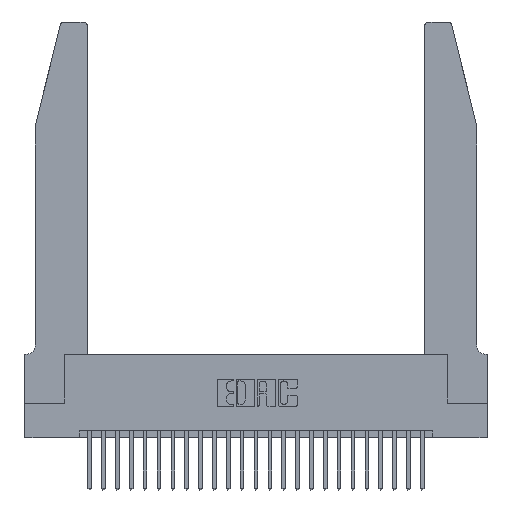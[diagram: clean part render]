
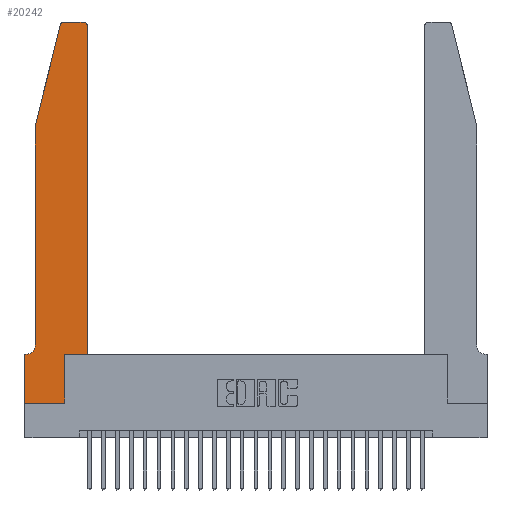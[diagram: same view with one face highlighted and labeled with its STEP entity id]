
A CAD part, top view. The second image highlights one B-rep face of the part: STEP entity #20242.
In plain terms, the highlighted planar face has unit normal (0, 0, 1).
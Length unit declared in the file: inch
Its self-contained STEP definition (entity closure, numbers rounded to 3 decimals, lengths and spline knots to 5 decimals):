
#42 = VECTOR ( 'NONE', #10206, 39.37008 ) ;
#264 = EDGE_CURVE ( 'NONE', #20774, #3971, #15840, .T. ) ;
#722 = FACE_OUTER_BOUND ( 'NONE', #21605, .T. ) ;
#1321 = VERTEX_POINT ( 'NONE', #15586 ) ;
#1489 = ORIENTED_EDGE ( 'NONE', *, *, #1849, .T. ) ;
#1694 = CARTESIAN_POINT ( 'NONE',  ( 0.0755, 0.42, 0.37 ) ) ;
#1849 = EDGE_CURVE ( 'NONE', #12343, #19882, #25817, .T. ) ;
#2294 = VECTOR ( 'NONE', #11618, 39.37008 ) ;
#3103 = DIRECTION ( 'NONE',  ( -0.239, -0.971, 0. ) ) ;
#3318 = ORIENTED_EDGE ( 'NONE', *, *, #16579, .T. ) ;
#3641 = PLANE ( 'NONE',  #5466 ) ;
#3971 = VERTEX_POINT ( 'NONE', #19977 ) ;
#4010 = DIRECTION ( 'NONE',  ( 0., 0., -1. ) ) ;
#4791 = DIRECTION ( 'NONE',  ( 0., 0., 1. ) ) ;
#4802 = EDGE_CURVE ( 'NONE', #21981, #8724, #15599, .T. ) ;
#4839 = VECTOR ( 'NONE', #3103, 39.37008 ) ;
#5466 = AXIS2_PLACEMENT_3D ( 'NONE', #18116, #5812, #20136 ) ;
#5775 = CARTESIAN_POINT ( 'NONE',  ( 0.2605, 2.75, 0.37 ) ) ;
#5780 = CARTESIAN_POINT ( 'NONE',  ( 0.25487, 2.72718, 0.37 ) ) ;
#5812 = DIRECTION ( 'NONE',  ( 0., 0., 1. ) ) ;
#5871 = EDGE_CURVE ( 'NONE', #24261, #24541, #8720, .T. ) ;
#5968 = DIRECTION ( 'NONE',  ( 0., -1., 0. ) ) ;
#6726 = CARTESIAN_POINT ( 'NONE',  ( 0.2865, 0.35, 0.37 ) ) ;
#6955 = EDGE_CURVE ( 'NONE', #3971, #21981, #16311, .T. ) ;
#7333 = EDGE_CURVE ( 'NONE', #25424, #12343, #23529, .T. ) ;
#7605 = CARTESIAN_POINT ( 'NONE',  ( 0.4205, 2.72, 0.37 ) ) ;
#8321 = DIRECTION ( 'NONE',  ( 0., -1., 0. ) ) ;
#8660 = CARTESIAN_POINT ( 'NONE',  ( 0.2865, 0., 0.37 ) ) ;
#8720 = CIRCLE ( 'NONE', #15561, 0.03 ) ;
#8724 = VERTEX_POINT ( 'NONE', #15977 ) ;
#8924 = AXIS2_PLACEMENT_3D ( 'NONE', #17145, #4791, #19156 ) ;
#9358 = VECTOR ( 'NONE', #16210, 39.37008 ) ;
#9700 = DIRECTION ( 'NONE',  ( 1., 0., 0. ) ) ;
#9787 = LINE ( 'NONE', #10392, #19938 ) ;
#10111 = EDGE_CURVE ( 'NONE', #20518, #25424, #9787, .T. ) ;
#10206 = DIRECTION ( 'NONE',  ( 0., 1., 0. ) ) ;
#10392 = CARTESIAN_POINT ( 'NONE',  ( 0., 0., 0.37 ) ) ;
#10727 = LINE ( 'NONE', #22314, #42 ) ;
#10774 = ORIENTED_EDGE ( 'NONE', *, *, #264, .T. ) ;
#11618 = DIRECTION ( 'NONE',  ( 1., 0., 0. ) ) ;
#12009 = VECTOR ( 'NONE', #25819, 39.37008 ) ;
#12221 = CARTESIAN_POINT ( 'NONE',  ( 0.2865, 0.35, 0.37 ) ) ;
#12343 = VERTEX_POINT ( 'NONE', #8660 ) ;
#12423 = CARTESIAN_POINT ( 'NONE',  ( 0.4505, 2.72, 0.37 ) ) ;
#12628 = LINE ( 'NONE', #23805, #12009 ) ;
#13145 = ORIENTED_EDGE ( 'NONE', *, *, #10111, .T. ) ;
#13219 = CARTESIAN_POINT ( 'NONE',  ( 0.4505, 0.35, 0.37 ) ) ;
#13655 = ORIENTED_EDGE ( 'NONE', *, *, #5871, .T. ) ;
#15008 = ORIENTED_EDGE ( 'NONE', *, *, #15850, .T. ) ;
#15404 = LINE ( 'NONE', #26222, #9358 ) ;
#15561 = AXIS2_PLACEMENT_3D ( 'NONE', #7605, #21805, #9700 ) ;
#15586 = CARTESIAN_POINT ( 'NONE',  ( 0.284, 2.75, 0.37 ) ) ;
#15599 = CIRCLE ( 'NONE', #22468, 0.07 ) ;
#15840 = LINE ( 'NONE', #24064, #4839 ) ;
#15850 = EDGE_CURVE ( 'NONE', #24541, #1321, #22457, .T. ) ;
#15977 = CARTESIAN_POINT ( 'NONE',  ( 0.0055, 0.35, 0.37 ) ) ;
#16210 = DIRECTION ( 'NONE',  ( -1., 0., 0. ) ) ;
#16311 = LINE ( 'NONE', #20290, #26364 ) ;
#16410 = CARTESIAN_POINT ( 'NONE',  ( 0.0055, 0.42, 0.37 ) ) ;
#16579 = EDGE_CURVE ( 'NONE', #17155, #24261, #10727, .T. ) ;
#16741 = EDGE_CURVE ( 'NONE', #1321, #20774, #23025, .T. ) ;
#16974 = EDGE_CURVE ( 'NONE', #19882, #17155, #12628, .T. ) ;
#17027 = CARTESIAN_POINT ( 'NONE',  ( 0., 0.35, 0.37 ) ) ;
#17122 = VECTOR ( 'NONE', #22083, 39.37008 ) ;
#17145 = CARTESIAN_POINT ( 'NONE',  ( 0.284, 2.72, 0.37 ) ) ;
#17155 = VERTEX_POINT ( 'NONE', #13219 ) ;
#17204 = ORIENTED_EDGE ( 'NONE', *, *, #7333, .T. ) ;
#18116 = CARTESIAN_POINT ( 'NONE',  ( 0., 0.35, 0.37 ) ) ;
#18312 = ORIENTED_EDGE ( 'NONE', *, *, #4802, .T. ) ;
#18446 = DIRECTION ( 'NONE',  ( -1., 0., 0. ) ) ;
#18837 = ORIENTED_EDGE ( 'NONE', *, *, #16741, .T. ) ;
#19009 = ORIENTED_EDGE ( 'NONE', *, *, #20791, .T. ) ;
#19156 = DIRECTION ( 'NONE',  ( 1., 0., 0. ) ) ;
#19882 = VERTEX_POINT ( 'NONE', #12221 ) ;
#19938 = VECTOR ( 'NONE', #8321, 39.37008 ) ;
#19977 = CARTESIAN_POINT ( 'NONE',  ( 0.0755, 2., 0.37 ) ) ;
#20136 = DIRECTION ( 'NONE',  ( 1., 0., 0. ) ) ;
#20242 = ADVANCED_FACE ( 'NONE', ( #722 ), #3641, .T. ) ;
#20290 = CARTESIAN_POINT ( 'NONE',  ( 0.0755, 2., 0.37 ) ) ;
#20518 = VERTEX_POINT ( 'NONE', #17027 ) ;
#20774 = VERTEX_POINT ( 'NONE', #5780 ) ;
#20791 = EDGE_CURVE ( 'NONE', #8724, #20518, #15404, .T. ) ;
#21605 = EDGE_LOOP ( 'NONE', ( #15008, #18837, #10774, #26608, #18312, #19009, #13145, #17204, #1489, #24441, #3318, #13655 ) ) ;
#21655 = CARTESIAN_POINT ( 'NONE',  ( 0., 0., 0.37 ) ) ;
#21805 = DIRECTION ( 'NONE',  ( 0., 0., 1. ) ) ;
#21956 = DIRECTION ( 'NONE',  ( 0., 1., 0. ) ) ;
#21981 = VERTEX_POINT ( 'NONE', #1694 ) ;
#22083 = DIRECTION ( 'NONE',  ( -1., 0., 0. ) ) ;
#22314 = CARTESIAN_POINT ( 'NONE',  ( 0.4505, 0.35, 0.37 ) ) ;
#22457 = LINE ( 'NONE', #5775, #17122 ) ;
#22468 = AXIS2_PLACEMENT_3D ( 'NONE', #16410, #4010, #18446 ) ;
#22751 = CARTESIAN_POINT ( 'NONE',  ( 0., 0., 0.37 ) ) ;
#23025 = CIRCLE ( 'NONE', #8924, 0.03 ) ;
#23529 = LINE ( 'NONE', #21655, #2294 ) ;
#23805 = CARTESIAN_POINT ( 'NONE',  ( 0.4505, 0.35, 0.37 ) ) ;
#23956 = CARTESIAN_POINT ( 'NONE',  ( 0.4205, 2.75, 0.37 ) ) ;
#24064 = CARTESIAN_POINT ( 'NONE',  ( 0.0755, 2., 0.37 ) ) ;
#24261 = VERTEX_POINT ( 'NONE', #12423 ) ;
#24441 = ORIENTED_EDGE ( 'NONE', *, *, #16974, .T. ) ;
#24541 = VERTEX_POINT ( 'NONE', #23956 ) ;
#25182 = VECTOR ( 'NONE', #21956, 39.37008 ) ;
#25424 = VERTEX_POINT ( 'NONE', #22751 ) ;
#25817 = LINE ( 'NONE', #6726, #25182 ) ;
#25819 = DIRECTION ( 'NONE',  ( 1., 0., 0. ) ) ;
#26222 = CARTESIAN_POINT ( 'NONE',  ( 0.0755, 0.35, 0.37 ) ) ;
#26364 = VECTOR ( 'NONE', #5968, 39.37008 ) ;
#26608 = ORIENTED_EDGE ( 'NONE', *, *, #6955, .T. ) ;
